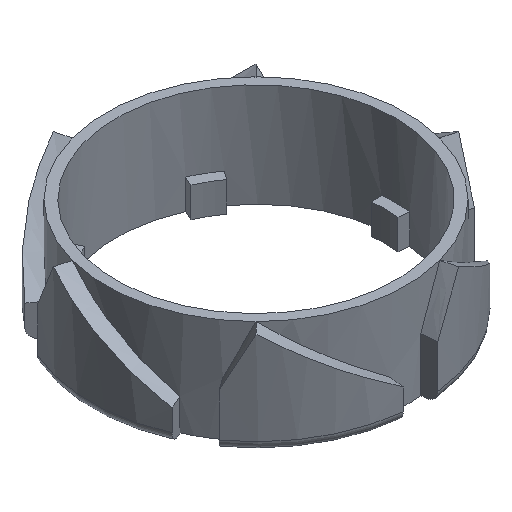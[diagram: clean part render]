
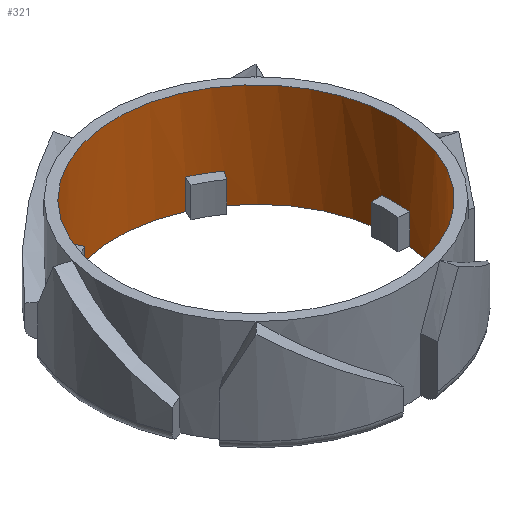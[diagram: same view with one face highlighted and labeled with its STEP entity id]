
A CAD part, isometric view. The second image highlights one B-rep face of the part: STEP entity #321.
In plain terms, the highlighted cylindrical face has radius 27.1 mm (diameter 54.2 mm), a full revolution.
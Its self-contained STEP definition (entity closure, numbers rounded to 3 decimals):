
#73=CARTESIAN_POINT('',(15.852,21.98,5.8));
#74=VERTEX_POINT('',#73);
#75=CARTESIAN_POINT('',(15.852,21.98,0.0));
#76=VERTEX_POINT('',#75);
#77=CARTESIAN_POINT('',(15.852,21.98,5.8));
#78=DIRECTION('',(0.0,0.0,-1.0));
#79=VECTOR('',#78,5.8);
#80=LINE('',#77,#79);
#81=EDGE_CURVE('',#74,#76,#80,.T.);
#108=CARTESIAN_POINT('',(0.0,0.0,0.0));
#109=DIRECTION('',(0.0,0.0,1.0));
#110=DIRECTION('',(-1.0,0.0,0.0));
#111=AXIS2_PLACEMENT_3D('',#108,#109,#110);
#112=CYLINDRICAL_SURFACE('',#111,27.1);
#113=CARTESIAN_POINT('',(27.1,0.,20.0));
#114=VERTEX_POINT('',#113);
#115=CARTESIAN_POINT('',(0.0,0.0,20.0));
#116=DIRECTION('',(0.0,0.0,-1.0));
#117=DIRECTION('',(-1.0,0.0,0.0));
#118=AXIS2_PLACEMENT_3D('',#115,#116,#117);
#119=CIRCLE('',#118,27.1);
#120=EDGE_CURVE('',#114,#114,#119,.T.);
#121=ORIENTED_EDGE('',*,*,#120,.F.);
#122=EDGE_LOOP('',(#121));
#123=FACE_OUTER_BOUND('',#122,.T.);
#124=CARTESIAN_POINT('',(11.109,24.718,5.8));
#125=VERTEX_POINT('',#124);
#126=CARTESIAN_POINT('',(0.0,0.0,5.8));
#127=DIRECTION('',(0.0,0.0,-1.0));
#128=DIRECTION('',(-1.0,0.0,0.0));
#129=AXIS2_PLACEMENT_3D('',#126,#127,#128);
#130=CIRCLE('',#129,27.1);
#131=EDGE_CURVE('',#125,#74,#130,.T.);
#132=ORIENTED_EDGE('',*,*,#131,.T.);
#133=ORIENTED_EDGE('',*,*,#81,.T.);
#134=CARTESIAN_POINT('',(26.961,2.739,0.0));
#135=VERTEX_POINT('',#134);
#136=CARTESIAN_POINT('',(0.0,0.0,0.0));
#137=DIRECTION('',(0.0,0.0,1.0));
#138=DIRECTION('',(-1.0,0.0,0.0));
#139=AXIS2_PLACEMENT_3D('',#136,#137,#138);
#140=CIRCLE('',#139,27.1);
#141=EDGE_CURVE('',#135,#76,#140,.T.);
#142=ORIENTED_EDGE('',*,*,#141,.F.);
#143=CARTESIAN_POINT('',(26.961,2.739,5.8));
#144=VERTEX_POINT('',#143);
#145=CARTESIAN_POINT('',(26.961,2.739,0.0));
#146=DIRECTION('',(0.0,0.0,1.0));
#147=VECTOR('',#146,5.8);
#148=LINE('',#145,#147);
#149=EDGE_CURVE('',#135,#144,#148,.T.);
#150=ORIENTED_EDGE('',*,*,#149,.T.);
#151=CARTESIAN_POINT('',(26.961,-2.739,5.8));
#152=VERTEX_POINT('',#151);
#153=CARTESIAN_POINT('',(0.0,0.0,5.8));
#154=DIRECTION('',(0.0,0.0,-1.0));
#155=DIRECTION('',(-1.0,0.0,0.0));
#156=AXIS2_PLACEMENT_3D('',#153,#154,#155);
#157=CIRCLE('',#156,27.1);
#158=EDGE_CURVE('',#144,#152,#157,.T.);
#159=ORIENTED_EDGE('',*,*,#158,.T.);
#160=CARTESIAN_POINT('',(26.961,-2.739,0.0));
#161=VERTEX_POINT('',#160);
#162=CARTESIAN_POINT('',(26.961,-2.739,5.8));
#163=DIRECTION('',(0.0,0.0,-1.0));
#164=VECTOR('',#163,5.8);
#165=LINE('',#162,#164);
#166=EDGE_CURVE('',#152,#161,#165,.T.);
#167=ORIENTED_EDGE('',*,*,#166,.T.);
#168=CARTESIAN_POINT('',(15.852,-21.98,0.0));
#169=VERTEX_POINT('',#168);
#170=CARTESIAN_POINT('',(0.0,0.0,0.0));
#171=DIRECTION('',(0.0,0.0,1.0));
#172=DIRECTION('',(-1.0,0.0,0.0));
#173=AXIS2_PLACEMENT_3D('',#170,#171,#172);
#174=CIRCLE('',#173,27.1);
#175=EDGE_CURVE('',#169,#161,#174,.T.);
#176=ORIENTED_EDGE('',*,*,#175,.F.);
#177=CARTESIAN_POINT('',(15.852,-21.98,5.8));
#178=VERTEX_POINT('',#177);
#179=CARTESIAN_POINT('',(15.852,-21.98,0.0));
#180=DIRECTION('',(0.0,0.0,1.0));
#181=VECTOR('',#180,5.8);
#182=LINE('',#179,#181);
#183=EDGE_CURVE('',#169,#178,#182,.T.);
#184=ORIENTED_EDGE('',*,*,#183,.T.);
#185=CARTESIAN_POINT('',(11.109,-24.718,5.8));
#186=VERTEX_POINT('',#185);
#187=CARTESIAN_POINT('',(0.0,0.0,5.8));
#188=DIRECTION('',(0.0,0.0,-1.0));
#189=DIRECTION('',(-1.0,0.0,0.0));
#190=AXIS2_PLACEMENT_3D('',#187,#188,#189);
#191=CIRCLE('',#190,27.1);
#192=EDGE_CURVE('',#178,#186,#191,.T.);
#193=ORIENTED_EDGE('',*,*,#192,.T.);
#194=CARTESIAN_POINT('',(11.109,-24.718,0.0));
#195=VERTEX_POINT('',#194);
#196=CARTESIAN_POINT('',(11.109,-24.718,5.8));
#197=DIRECTION('',(0.0,0.0,-1.0));
#198=VECTOR('',#197,5.8);
#199=LINE('',#196,#198);
#200=EDGE_CURVE('',#186,#195,#199,.T.);
#201=ORIENTED_EDGE('',*,*,#200,.T.);
#202=CARTESIAN_POINT('',(-11.109,-24.718,0.0));
#203=VERTEX_POINT('',#202);
#204=CARTESIAN_POINT('',(0.0,0.0,0.0));
#205=DIRECTION('',(0.0,0.0,1.0));
#206=DIRECTION('',(-1.0,0.0,0.0));
#207=AXIS2_PLACEMENT_3D('',#204,#205,#206);
#208=CIRCLE('',#207,27.1);
#209=EDGE_CURVE('',#203,#195,#208,.T.);
#210=ORIENTED_EDGE('',*,*,#209,.F.);
#211=CARTESIAN_POINT('',(-11.109,-24.718,5.8));
#212=VERTEX_POINT('',#211);
#213=CARTESIAN_POINT('',(-11.109,-24.718,0.0));
#214=DIRECTION('',(0.0,0.0,1.0));
#215=VECTOR('',#214,5.8);
#216=LINE('',#213,#215);
#217=EDGE_CURVE('',#203,#212,#216,.T.);
#218=ORIENTED_EDGE('',*,*,#217,.T.);
#219=CARTESIAN_POINT('',(-15.852,-21.98,5.8));
#220=VERTEX_POINT('',#219);
#221=CARTESIAN_POINT('',(0.0,0.0,5.8));
#222=DIRECTION('',(0.0,0.0,-1.0));
#223=DIRECTION('',(-1.0,0.0,0.0));
#224=AXIS2_PLACEMENT_3D('',#221,#222,#223);
#225=CIRCLE('',#224,27.1);
#226=EDGE_CURVE('',#212,#220,#225,.T.);
#227=ORIENTED_EDGE('',*,*,#226,.T.);
#228=CARTESIAN_POINT('',(-15.852,-21.98,0.0));
#229=VERTEX_POINT('',#228);
#230=CARTESIAN_POINT('',(-15.852,-21.98,5.8));
#231=DIRECTION('',(0.0,0.0,-1.0));
#232=VECTOR('',#231,5.8);
#233=LINE('',#230,#232);
#234=EDGE_CURVE('',#220,#229,#233,.T.);
#235=ORIENTED_EDGE('',*,*,#234,.T.);
#236=CARTESIAN_POINT('',(-26.961,-2.739,0.0));
#237=VERTEX_POINT('',#236);
#238=CARTESIAN_POINT('',(0.0,0.0,0.0));
#239=DIRECTION('',(0.0,0.0,1.0));
#240=DIRECTION('',(-1.0,0.0,0.0));
#241=AXIS2_PLACEMENT_3D('',#238,#239,#240);
#242=CIRCLE('',#241,27.1);
#243=EDGE_CURVE('',#237,#229,#242,.T.);
#244=ORIENTED_EDGE('',*,*,#243,.F.);
#245=CARTESIAN_POINT('',(-26.961,-2.739,5.8));
#246=VERTEX_POINT('',#245);
#247=CARTESIAN_POINT('',(-26.961,-2.739,0.0));
#248=DIRECTION('',(0.0,0.0,1.0));
#249=VECTOR('',#248,5.8);
#250=LINE('',#247,#249);
#251=EDGE_CURVE('',#237,#246,#250,.T.);
#252=ORIENTED_EDGE('',*,*,#251,.T.);
#253=CARTESIAN_POINT('',(-26.961,2.739,5.8));
#254=VERTEX_POINT('',#253);
#255=CARTESIAN_POINT('',(0.0,0.0,5.8));
#256=DIRECTION('',(0.0,0.0,-1.0));
#257=DIRECTION('',(-1.0,0.0,0.0));
#258=AXIS2_PLACEMENT_3D('',#255,#256,#257);
#259=CIRCLE('',#258,27.1);
#260=EDGE_CURVE('',#246,#254,#259,.T.);
#261=ORIENTED_EDGE('',*,*,#260,.T.);
#262=CARTESIAN_POINT('',(-26.961,2.739,0.0));
#263=VERTEX_POINT('',#262);
#264=CARTESIAN_POINT('',(-26.961,2.739,5.8));
#265=DIRECTION('',(0.0,0.0,-1.0));
#266=VECTOR('',#265,5.8);
#267=LINE('',#264,#266);
#268=EDGE_CURVE('',#254,#263,#267,.T.);
#269=ORIENTED_EDGE('',*,*,#268,.T.);
#270=CARTESIAN_POINT('',(-15.852,21.98,0.0));
#271=VERTEX_POINT('',#270);
#272=CARTESIAN_POINT('',(0.0,0.0,0.0));
#273=DIRECTION('',(0.0,0.0,1.0));
#274=DIRECTION('',(-1.0,0.0,0.0));
#275=AXIS2_PLACEMENT_3D('',#272,#273,#274);
#276=CIRCLE('',#275,27.1);
#277=EDGE_CURVE('',#271,#263,#276,.T.);
#278=ORIENTED_EDGE('',*,*,#277,.F.);
#279=CARTESIAN_POINT('',(-15.852,21.98,5.8));
#280=VERTEX_POINT('',#279);
#281=CARTESIAN_POINT('',(-15.852,21.98,0.0));
#282=DIRECTION('',(0.0,0.0,1.0));
#283=VECTOR('',#282,5.8);
#284=LINE('',#281,#283);
#285=EDGE_CURVE('',#271,#280,#284,.T.);
#286=ORIENTED_EDGE('',*,*,#285,.T.);
#287=CARTESIAN_POINT('',(-11.109,24.718,5.8));
#288=VERTEX_POINT('',#287);
#289=CARTESIAN_POINT('',(0.0,0.0,5.8));
#290=DIRECTION('',(0.0,0.0,-1.0));
#291=DIRECTION('',(-1.0,0.0,0.0));
#292=AXIS2_PLACEMENT_3D('',#289,#290,#291);
#293=CIRCLE('',#292,27.1);
#294=EDGE_CURVE('',#280,#288,#293,.T.);
#295=ORIENTED_EDGE('',*,*,#294,.T.);
#296=CARTESIAN_POINT('',(-11.109,24.718,0.0));
#297=VERTEX_POINT('',#296);
#298=CARTESIAN_POINT('',(-11.109,24.718,5.8));
#299=DIRECTION('',(0.0,0.0,-1.0));
#300=VECTOR('',#299,5.8);
#301=LINE('',#298,#300);
#302=EDGE_CURVE('',#288,#297,#301,.T.);
#303=ORIENTED_EDGE('',*,*,#302,.T.);
#304=CARTESIAN_POINT('',(11.109,24.718,0.0));
#305=VERTEX_POINT('',#304);
#306=CARTESIAN_POINT('',(0.0,0.0,0.0));
#307=DIRECTION('',(0.0,0.0,1.0));
#308=DIRECTION('',(-1.0,0.0,0.0));
#309=AXIS2_PLACEMENT_3D('',#306,#307,#308);
#310=CIRCLE('',#309,27.1);
#311=EDGE_CURVE('',#305,#297,#310,.T.);
#312=ORIENTED_EDGE('',*,*,#311,.F.);
#313=CARTESIAN_POINT('',(11.109,24.718,0.0));
#314=DIRECTION('',(0.0,0.0,1.0));
#315=VECTOR('',#314,5.8);
#316=LINE('',#313,#315);
#317=EDGE_CURVE('',#305,#125,#316,.T.);
#318=ORIENTED_EDGE('',*,*,#317,.T.);
#319=EDGE_LOOP('',(#132,#133,#142,#150,#159,#167,#176,#184,#193,#201,#210,#218,#227,#235,#244,#252,#261,#269,#278,#286,#295,#303,#312,#318));
#320=FACE_BOUND('',#319,.T.);
#321=ADVANCED_FACE('',(#123,#320),#112,.F.);
